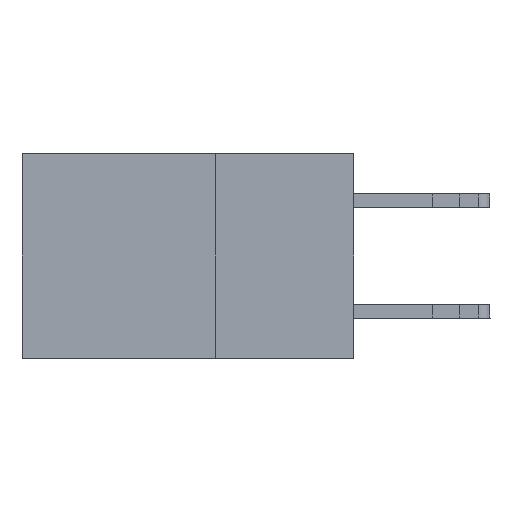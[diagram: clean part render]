
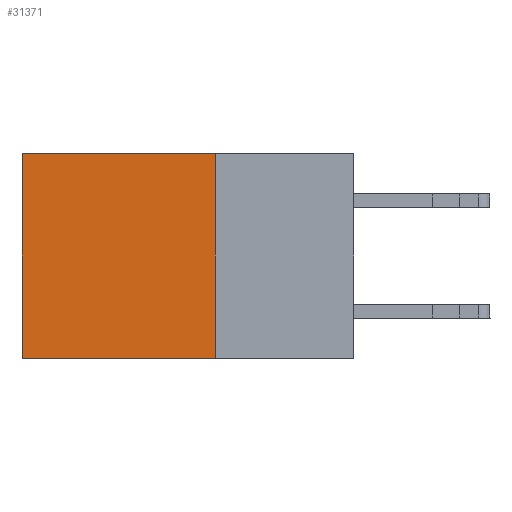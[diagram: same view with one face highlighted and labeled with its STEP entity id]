
A CAD part, left-side view. The second image highlights one B-rep face of the part: STEP entity #31371.
In plain terms, the highlighted planar face has unit normal (-1, 0, 0).
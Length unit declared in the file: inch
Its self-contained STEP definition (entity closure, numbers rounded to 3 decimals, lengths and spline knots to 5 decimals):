
#899 = LINE ( 'NONE', #27604, #28553 ) ;
#2126 = DIRECTION ( 'NONE',  ( 0., 1., 0. ) ) ;
#2527 = VERTEX_POINT ( 'NONE', #24452 ) ;
#3921 = VERTEX_POINT ( 'NONE', #5438 ) ;
#4393 = ORIENTED_EDGE ( 'NONE', *, *, #26504, .F. ) ;
#5174 = CARTESIAN_POINT ( 'NONE',  ( 0.2875, 0.6, 0. ) ) ;
#5438 = CARTESIAN_POINT ( 'NONE',  ( 0.2875, 0.6, -0.37 ) ) ;
#5506 = CARTESIAN_POINT ( 'NONE',  ( 0.2875, 0.25, -0.37 ) ) ;
#8163 = DIRECTION ( 'NONE',  ( 0., 0., -1. ) ) ;
#9224 = VECTOR ( 'NONE', #8163, 39.37008 ) ;
#9910 = ORIENTED_EDGE ( 'NONE', *, *, #14226, .T. ) ;
#10839 = CARTESIAN_POINT ( 'NONE',  ( 0.2875, 0.6, 0. ) ) ;
#11288 = CARTESIAN_POINT ( 'NONE',  ( 0.2875, 0.25, 0. ) ) ;
#12464 = CARTESIAN_POINT ( 'NONE',  ( 0.2875, 0.25, 0. ) ) ;
#14226 = EDGE_CURVE ( 'NONE', #22815, #3921, #34143, .T. ) ;
#16102 = AXIS2_PLACEMENT_3D ( 'NONE', #12464, #23916, #35738 ) ;
#18902 = DIRECTION ( 'NONE',  ( 0., 0., -1. ) ) ;
#20207 = CARTESIAN_POINT ( 'NONE',  ( 0.2875, 0.25, -0.37 ) ) ;
#20580 = ORIENTED_EDGE ( 'NONE', *, *, #33017, .T. ) ;
#21645 = PLANE ( 'NONE',  #16102 ) ;
#21778 = ORIENTED_EDGE ( 'NONE', *, *, #25181, .F. ) ;
#22815 = VERTEX_POINT ( 'NONE', #5174 ) ;
#23916 = DIRECTION ( 'NONE',  ( 1., 0., 0. ) ) ;
#24452 = CARTESIAN_POINT ( 'NONE',  ( 0.2875, 0.25, 0. ) ) ;
#25181 = EDGE_CURVE ( 'NONE', #27974, #3921, #27279, .T. ) ;
#26133 = DIRECTION ( 'NONE',  ( 0., 1., 0. ) ) ;
#26504 = EDGE_CURVE ( 'NONE', #2527, #27974, #899, .T. ) ;
#27279 = LINE ( 'NONE', #5506, #27747 ) ;
#27604 = CARTESIAN_POINT ( 'NONE',  ( 0.2875, 0.25, 0. ) ) ;
#27747 = VECTOR ( 'NONE', #26133, 39.37008 ) ;
#27974 = VERTEX_POINT ( 'NONE', #20207 ) ;
#28553 = VECTOR ( 'NONE', #18902, 39.37008 ) ;
#30104 = VECTOR ( 'NONE', #2126, 39.37008 ) ;
#31371 = ADVANCED_FACE ( 'NONE', ( #35291 ), #21645, .F. ) ;
#33017 = EDGE_CURVE ( 'NONE', #2527, #22815, #37924, .T. ) ;
#34143 = LINE ( 'NONE', #10839, #9224 ) ;
#35291 = FACE_OUTER_BOUND ( 'NONE', #36424, .T. ) ;
#35738 = DIRECTION ( 'NONE',  ( 0., 0., -1. ) ) ;
#36424 = EDGE_LOOP ( 'NONE', ( #9910, #21778, #4393, #20580 ) ) ;
#37924 = LINE ( 'NONE', #11288, #30104 ) ;
